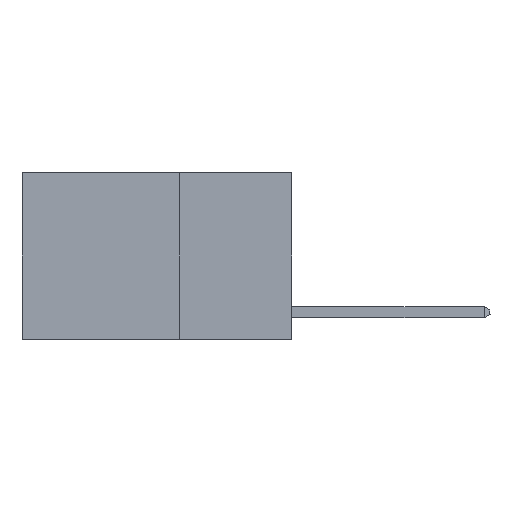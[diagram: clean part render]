
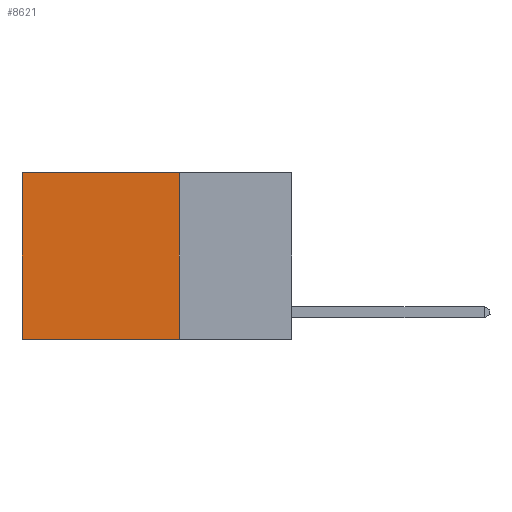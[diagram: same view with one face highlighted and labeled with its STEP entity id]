
A CAD part, left-side view. The second image highlights one B-rep face of the part: STEP entity #8621.
In plain terms, the highlighted planar face has unit normal (-1, 0, 0).
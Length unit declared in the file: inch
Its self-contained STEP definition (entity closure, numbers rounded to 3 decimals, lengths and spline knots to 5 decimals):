
#127 = CARTESIAN_POINT ( 'NONE',  ( 0.2625, 0.25, 0. ) ) ;
#396 = CARTESIAN_POINT ( 'NONE',  ( 0.2625, 0.6, 0. ) ) ;
#405 = ORIENTED_EDGE ( 'NONE', *, *, #17556, .T. ) ;
#1453 = LINE ( 'NONE', #127, #5171 ) ;
#1874 = EDGE_CURVE ( 'NONE', #3947, #8673, #3348, .T. ) ;
#3042 = DIRECTION ( 'NONE',  ( 0., 0., -1. ) ) ;
#3348 = LINE ( 'NONE', #11036, #6570 ) ;
#3947 = VERTEX_POINT ( 'NONE', #396 ) ;
#4755 = DIRECTION ( 'NONE',  ( 0., 0., -1. ) ) ;
#4814 = VECTOR ( 'NONE', #3042, 39.37008 ) ;
#4823 = EDGE_CURVE ( 'NONE', #15548, #8673, #12672, .T. ) ;
#5171 = VECTOR ( 'NONE', #15729, 39.37008 ) ;
#6500 = ORIENTED_EDGE ( 'NONE', *, *, #4823, .F. ) ;
#6570 = VECTOR ( 'NONE', #4755, 39.37008 ) ;
#8168 = FACE_OUTER_BOUND ( 'NONE', #14855, .T. ) ;
#8417 = EDGE_CURVE ( 'NONE', #14518, #15548, #16865, .T. ) ;
#8621 = ADVANCED_FACE ( 'NONE', ( #8168 ), #18795, .F. ) ;
#8673 = VERTEX_POINT ( 'NONE', #15017 ) ;
#10916 = VECTOR ( 'NONE', #11143, 39.37008 ) ;
#11032 = CARTESIAN_POINT ( 'NONE',  ( 0.2625, 0.25, 0. ) ) ;
#11036 = CARTESIAN_POINT ( 'NONE',  ( 0.2625, 0.6, 0. ) ) ;
#11143 = DIRECTION ( 'NONE',  ( 0., 1., 0. ) ) ;
#12672 = LINE ( 'NONE', #18899, #10916 ) ;
#13904 = CARTESIAN_POINT ( 'NONE',  ( 0.2625, 0.25, 0. ) ) ;
#14518 = VERTEX_POINT ( 'NONE', #13904 ) ;
#14855 = EDGE_LOOP ( 'NONE', ( #15787, #6500, #17984, #405 ) ) ;
#15017 = CARTESIAN_POINT ( 'NONE',  ( 0.2625, 0.6, -0.37 ) ) ;
#15548 = VERTEX_POINT ( 'NONE', #17880 ) ;
#15729 = DIRECTION ( 'NONE',  ( 0., 1., 0. ) ) ;
#15755 = DIRECTION ( 'NONE',  ( 1., 0., 0. ) ) ;
#15787 = ORIENTED_EDGE ( 'NONE', *, *, #1874, .T. ) ;
#16865 = LINE ( 'NONE', #17173, #4814 ) ;
#16942 = AXIS2_PLACEMENT_3D ( 'NONE', #11032, #15755, #19097 ) ;
#17173 = CARTESIAN_POINT ( 'NONE',  ( 0.2625, 0.25, 0. ) ) ;
#17556 = EDGE_CURVE ( 'NONE', #14518, #3947, #1453, .T. ) ;
#17880 = CARTESIAN_POINT ( 'NONE',  ( 0.2625, 0.25, -0.37 ) ) ;
#17984 = ORIENTED_EDGE ( 'NONE', *, *, #8417, .F. ) ;
#18795 = PLANE ( 'NONE',  #16942 ) ;
#18899 = CARTESIAN_POINT ( 'NONE',  ( 0.2625, 0.25, -0.37 ) ) ;
#19097 = DIRECTION ( 'NONE',  ( 0., 0., -1. ) ) ;
